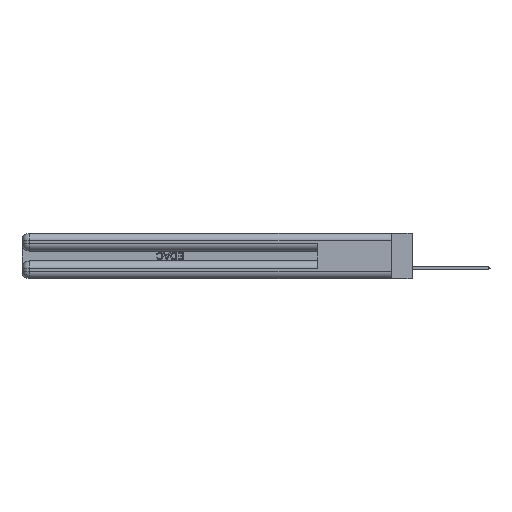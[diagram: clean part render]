
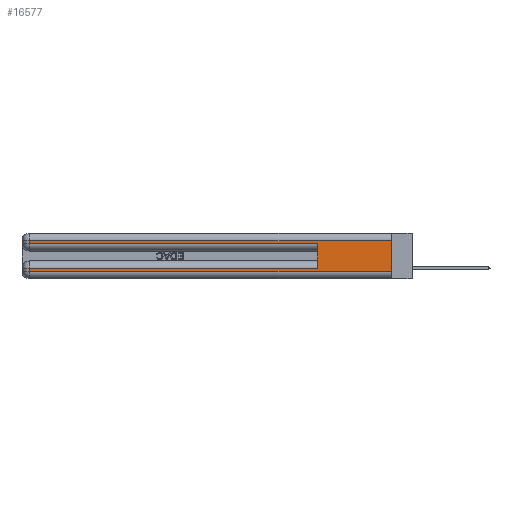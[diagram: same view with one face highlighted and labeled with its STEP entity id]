
A CAD part, left-side view. The second image highlights one B-rep face of the part: STEP entity #16577.
In plain terms, the highlighted planar face has unit normal (-1, 0, 0).
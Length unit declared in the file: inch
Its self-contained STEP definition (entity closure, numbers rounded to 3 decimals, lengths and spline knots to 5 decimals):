
#1063 = CARTESIAN_POINT ( 'NONE',  ( 0., 2.94, 0.085 ) ) ;
#1455 = ORIENTED_EDGE ( 'NONE', *, *, #29681, .T. ) ;
#1857 = LINE ( 'NONE', #40081, #28360 ) ;
#1913 = VECTOR ( 'NONE', #14807, 39.37008 ) ;
#3499 = DIRECTION ( 'NONE',  ( 0., 1., 0. ) ) ;
#4520 = LINE ( 'NONE', #44357, #1913 ) ;
#4842 = CARTESIAN_POINT ( 'NONE',  ( 0., 0., 0.285 ) ) ;
#6255 = LINE ( 'NONE', #35092, #13985 ) ;
#7272 = CARTESIAN_POINT ( 'NONE',  ( 0., 0., 0.085 ) ) ;
#7412 = VECTOR ( 'NONE', #42398, 39.37008 ) ;
#8072 = VECTOR ( 'NONE', #25978, 39.37008 ) ;
#9190 = DIRECTION ( 'NONE',  ( 0., 0., 1. ) ) ;
#9216 = VECTOR ( 'NONE', #3499, 39.37008 ) ;
#9901 = VERTEX_POINT ( 'NONE', #28873 ) ;
#10306 = DIRECTION ( 'NONE',  ( 0., 0., -1. ) ) ;
#13985 = VECTOR ( 'NONE', #10306, 39.37008 ) ;
#14807 = DIRECTION ( 'NONE',  ( 0., -1., 0. ) ) ;
#15956 = CARTESIAN_POINT ( 'NONE',  ( 0., 0., 0.06 ) ) ;
#16168 = CARTESIAN_POINT ( 'NONE',  ( 0., 2.94, 0.285 ) ) ;
#16577 = ADVANCED_FACE ( 'NONE', ( #44058 ), #37680, .F. ) ;
#16694 = CARTESIAN_POINT ( 'NONE',  ( 0., 2.94, 0.06 ) ) ;
#17033 = EDGE_CURVE ( 'NONE', #30210, #42117, #6255, .T. ) ;
#18129 = CARTESIAN_POINT ( 'NONE',  ( 0., 0.6, 0.085 ) ) ;
#18291 = VECTOR ( 'NONE', #9190, 39.37008 ) ;
#19121 = EDGE_LOOP ( 'NONE', ( #30488, #37150, #32522, #23200, #21874, #27628, #1455, #49869 ) ) ;
#21426 = EDGE_CURVE ( 'NONE', #49976, #42117, #4520, .T. ) ;
#21443 = AXIS2_PLACEMENT_3D ( 'NONE', #41507, #45719, #21591 ) ;
#21591 = DIRECTION ( 'NONE',  ( 0., 0., -1. ) ) ;
#21874 = ORIENTED_EDGE ( 'NONE', *, *, #40592, .F. ) ;
#23200 = ORIENTED_EDGE ( 'NONE', *, *, #48264, .T. ) ;
#24971 = LINE ( 'NONE', #4842, #39863 ) ;
#25978 = DIRECTION ( 'NONE',  ( 0., 1., 0. ) ) ;
#27307 = CARTESIAN_POINT ( 'NONE',  ( 0., 0.6, 0.285 ) ) ;
#27628 = ORIENTED_EDGE ( 'NONE', *, *, #33677, .T. ) ;
#28360 = VECTOR ( 'NONE', #52096, 39.37008 ) ;
#28873 = CARTESIAN_POINT ( 'NONE',  ( 0., 2.94, 0.31 ) ) ;
#29353 = LINE ( 'NONE', #34170, #18291 ) ;
#29681 = EDGE_CURVE ( 'NONE', #53463, #49976, #1857, .T. ) ;
#30210 = VERTEX_POINT ( 'NONE', #36500 ) ;
#30488 = ORIENTED_EDGE ( 'NONE', *, *, #17033, .F. ) ;
#30702 = LINE ( 'NONE', #30706, #8072 ) ;
#30706 = CARTESIAN_POINT ( 'NONE',  ( 0., 0., 0.31 ) ) ;
#32522 = ORIENTED_EDGE ( 'NONE', *, *, #39857, .T. ) ;
#33677 = EDGE_CURVE ( 'NONE', #43462, #53463, #36400, .T. ) ;
#34170 = CARTESIAN_POINT ( 'NONE',  ( 0., 0.6, 0.145 ) ) ;
#34551 = VERTEX_POINT ( 'NONE', #16168 ) ;
#34597 = LINE ( 'NONE', #50608, #7412 ) ;
#35092 = CARTESIAN_POINT ( 'NONE',  ( 0., 0., 0.37 ) ) ;
#36400 = LINE ( 'NONE', #7272, #9216 ) ;
#36500 = CARTESIAN_POINT ( 'NONE',  ( 0., 0., 0.31 ) ) ;
#37150 = ORIENTED_EDGE ( 'NONE', *, *, #42439, .T. ) ;
#37680 = PLANE ( 'NONE',  #21443 ) ;
#39857 = EDGE_CURVE ( 'NONE', #9901, #34551, #34597, .T. ) ;
#39863 = VECTOR ( 'NONE', #42071, 39.37008 ) ;
#40081 = CARTESIAN_POINT ( 'NONE',  ( 0., 2.94, 0.37 ) ) ;
#40592 = EDGE_CURVE ( 'NONE', #43462, #42024, #29353, .T. ) ;
#41507 = CARTESIAN_POINT ( 'NONE',  ( 0., 0., 0.37 ) ) ;
#42024 = VERTEX_POINT ( 'NONE', #27307 ) ;
#42071 = DIRECTION ( 'NONE',  ( 0., -1., 0. ) ) ;
#42117 = VERTEX_POINT ( 'NONE', #15956 ) ;
#42398 = DIRECTION ( 'NONE',  ( 0., 0., -1. ) ) ;
#42439 = EDGE_CURVE ( 'NONE', #30210, #9901, #30702, .T. ) ;
#43462 = VERTEX_POINT ( 'NONE', #18129 ) ;
#44058 = FACE_OUTER_BOUND ( 'NONE', #19121, .T. ) ;
#44357 = CARTESIAN_POINT ( 'NONE',  ( 0., 0., 0.06 ) ) ;
#45719 = DIRECTION ( 'NONE',  ( 1., 0., 0. ) ) ;
#48264 = EDGE_CURVE ( 'NONE', #34551, #42024, #24971, .T. ) ;
#49869 = ORIENTED_EDGE ( 'NONE', *, *, #21426, .T. ) ;
#49976 = VERTEX_POINT ( 'NONE', #16694 ) ;
#50608 = CARTESIAN_POINT ( 'NONE',  ( 0., 2.94, 0.37 ) ) ;
#52096 = DIRECTION ( 'NONE',  ( 0., 0., -1. ) ) ;
#53463 = VERTEX_POINT ( 'NONE', #1063 ) ;
